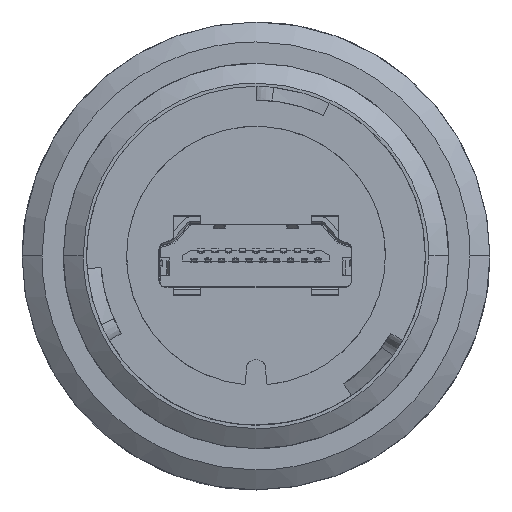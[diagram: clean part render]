
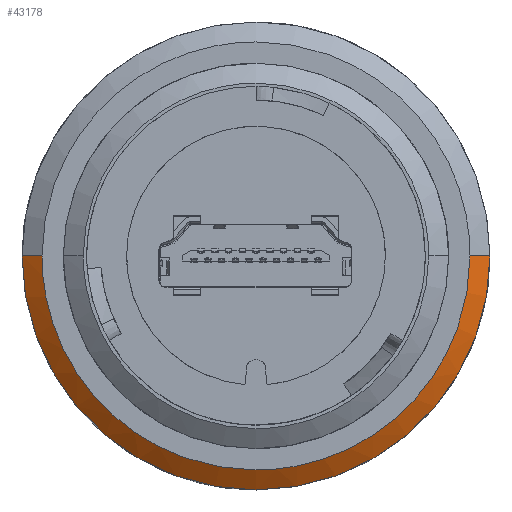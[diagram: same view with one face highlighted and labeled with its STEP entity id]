
A CAD part, top view. The second image highlights one B-rep face of the part: STEP entity #43178.
In plain terms, the highlighted conical face has half-angle 55.408 degrees and reference radius 17 mm.
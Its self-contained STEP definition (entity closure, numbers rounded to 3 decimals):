
#275 = CONICAL_SURFACE ( 'NONE', #16199, 17., 0.967 ) ;
#1208 = CARTESIAN_POINT ( 'NONE',  ( -13., -15.55, 0. ) ) ;
#1401 = CARTESIAN_POINT ( 'NONE',  ( -13., 0., -15.55 ) ) ;
#2434 = VERTEX_POINT ( 'NONE', #1401 ) ;
#3846 = CARTESIAN_POINT ( 'NONE',  ( -13., -2.035, -15.55 ) ) ;
#4165 = DIRECTION ( 'NONE',  ( 0., 0., 1. ) ) ;
#4554 = EDGE_CURVE ( 'NONE', #27924, #27990, #11954, .T. ) ;
#6435 = ORIENTED_EDGE ( 'NONE', *, *, #16587, .F. ) ;
#6588 = CARTESIAN_POINT ( 'NONE',  ( -13., 0., 15.55 ) ) ;
#7623 = CARTESIAN_POINT ( 'NONE',  ( -13., 0., -15.55 ) ) ;
#7756 = VERTEX_POINT ( 'NONE', #6588 ) ;
#8094 = CARTESIAN_POINT ( 'NONE',  ( -13., -12.435, -9.556 ) ) ;
#10659 = CARTESIAN_POINT ( 'NONE',  ( -13., -7.831, 13.587 ) ) ;
#11123 = CARTESIAN_POINT ( 'NONE',  ( -13., -15.55, 2.035 ) ) ;
#11422 = DIRECTION ( 'NONE',  ( -1., 0., 0. ) ) ;
#11954 = CIRCLE ( 'NONE', #18030, 17. ) ;
#12432 = ORIENTED_EDGE ( 'NONE', *, *, #15275, .T. ) ;
#14219 = CARTESIAN_POINT ( 'NONE',  ( -13., -9.556, 12.435 ) ) ;
#14463 = LINE ( 'NONE', #28945, #43684 ) ;
#15275 = EDGE_CURVE ( 'NONE', #15768, #7756, #24058, .T. ) ;
#15768 = VERTEX_POINT ( 'NONE', #30056 ) ;
#16031 = EDGE_CURVE ( 'NONE', #7756, #27990, #33042, .T. ) ;
#16199 = AXIS2_PLACEMENT_3D ( 'NONE', #34071, #22899, #4165 ) ;
#16587 = EDGE_CURVE ( 'NONE', #2434, #27924, #14463, .T. ) ;
#18030 = AXIS2_PLACEMENT_3D ( 'NONE', #33752, #11422, #29706 ) ;
#18365 = EDGE_LOOP ( 'NONE', ( #6435, #19423, #12432, #32794, #23136 ) ) ;
#19423 = ORIENTED_EDGE ( 'NONE', *, *, #23430, .T. ) ;
#21814 = CARTESIAN_POINT ( 'NONE',  ( -13., -4.07, 15.145 ) ) ;
#21824 = DIRECTION ( 'NONE',  ( -0.568, 0., -0.823 ) ) ;
#22345 = CARTESIAN_POINT ( 'NONE',  ( -13., -4.07, -15.145 ) ) ;
#22587 = CARTESIAN_POINT ( 'NONE',  ( -13., -15.145, -4.07 ) ) ;
#22899 = DIRECTION ( 'NONE',  ( -1., 0., 0. ) ) ;
#23136 = ORIENTED_EDGE ( 'NONE', *, *, #4554, .F. ) ;
#23241 = CARTESIAN_POINT ( 'NONE',  ( -14., 0., -17. ) ) ;
#23430 = EDGE_CURVE ( 'NONE', #2434, #15768, #35863, .T. ) ;
#23940 = VECTOR ( 'NONE', #25671, 1000. ) ;
#24058 = B_SPLINE_CURVE_WITH_KNOTS ( 'NONE', 3,
 ( #39617, #11123, #43415, #32973, #35592, #14219, #10659, #21814, #39015, #28467 ),
 .UNSPECIFIED., .F., .F.,
 ( 4, 2, 2, 2, 4 ),
 ( 0., 0.125, 0.25, 0.375, 0.5 ),
 .UNSPECIFIED. ) ;
#25671 = DIRECTION ( 'NONE',  ( -0.568, 0., 0.823 ) ) ;
#26376 = CARTESIAN_POINT ( 'NONE',  ( -13., -13.587, -7.831 ) ) ;
#27924 = VERTEX_POINT ( 'NONE', #23241 ) ;
#27990 = VERTEX_POINT ( 'NONE', #37047 ) ;
#28467 = CARTESIAN_POINT ( 'NONE',  ( -13., 0., 15.55 ) ) ;
#28945 = CARTESIAN_POINT ( 'NONE',  ( -14., 0., -17. ) ) ;
#29706 = DIRECTION ( 'NONE',  ( 0., 0., -1. ) ) ;
#30056 = CARTESIAN_POINT ( 'NONE',  ( -13., -15.55, 0. ) ) ;
#30276 = FACE_OUTER_BOUND ( 'NONE', #18365, .T. ) ;
#32794 = ORIENTED_EDGE ( 'NONE', *, *, #16031, .T. ) ;
#32973 = CARTESIAN_POINT ( 'NONE',  ( -13., -13.587, 7.831 ) ) ;
#33042 = LINE ( 'NONE', #33283, #23940 ) ;
#33283 = CARTESIAN_POINT ( 'NONE',  ( -14., 0., 17. ) ) ;
#33752 = CARTESIAN_POINT ( 'NONE',  ( -14., 0., 0. ) ) ;
#34071 = CARTESIAN_POINT ( 'NONE',  ( -14., 0., 0. ) ) ;
#35592 = CARTESIAN_POINT ( 'NONE',  ( -13., -12.435, 9.556 ) ) ;
#35863 = B_SPLINE_CURVE_WITH_KNOTS ( 'NONE', 3,
 ( #7623, #3846, #22345, #36839, #40639, #8094, #26376, #22587, #37081, #1208 ),
 .UNSPECIFIED., .F., .F.,
 ( 4, 2, 2, 2, 4 ),
 ( 0.5, 0.625, 0.75, 0.875, 1. ),
 .UNSPECIFIED. ) ;
#36839 = CARTESIAN_POINT ( 'NONE',  ( -13., -7.831, -13.587 ) ) ;
#37047 = CARTESIAN_POINT ( 'NONE',  ( -14., 0., 17. ) ) ;
#37081 = CARTESIAN_POINT ( 'NONE',  ( -13., -15.55, -2.035 ) ) ;
#39015 = CARTESIAN_POINT ( 'NONE',  ( -13., -2.035, 15.55 ) ) ;
#39617 = CARTESIAN_POINT ( 'NONE',  ( -13., -15.55, 0. ) ) ;
#40639 = CARTESIAN_POINT ( 'NONE',  ( -13., -9.556, -12.435 ) ) ;
#43178 = ADVANCED_FACE ( 'NONE', ( #30276 ), #275, .T. ) ;
#43415 = CARTESIAN_POINT ( 'NONE',  ( -13., -15.145, 4.07 ) ) ;
#43684 = VECTOR ( 'NONE', #21824, 1000. ) ;
